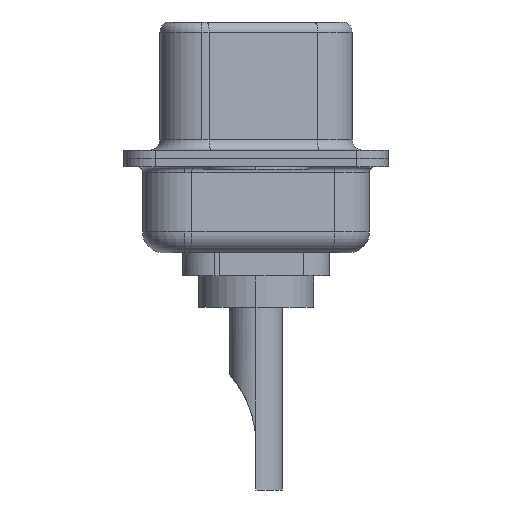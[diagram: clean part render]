
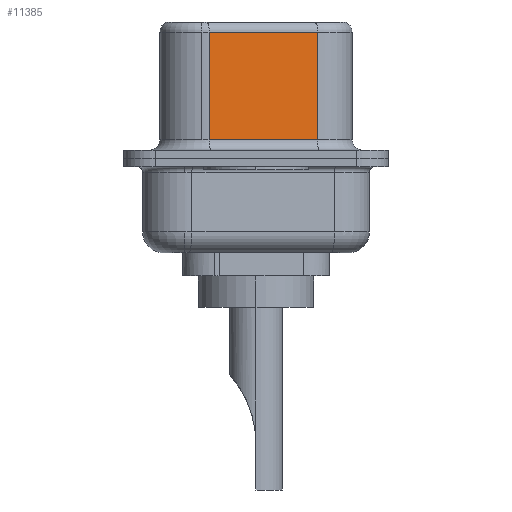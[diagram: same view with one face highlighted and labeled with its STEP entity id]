
A CAD part, left-side view. The second image highlights one B-rep face of the part: STEP entity #11385.
In plain terms, the highlighted planar face has unit normal (-0.985, -0.174, 0).
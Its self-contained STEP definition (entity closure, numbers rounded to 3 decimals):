
#25 = CARTESIAN_POINT ( 'NONE',  ( 4.585, -2.927, 6.02 ) ) ;
#292 = ORIENTED_EDGE ( 'NONE', *, *, #6385, .T. ) ;
#696 = AXIS2_PLACEMENT_3D ( 'NONE', #10534, #4823, #11581 ) ;
#2367 = CARTESIAN_POINT ( 'NONE',  ( 4.585, -2.927, 6.02 ) ) ;
#3522 = DIRECTION ( 'NONE',  ( 0., 0., -1. ) ) ;
#3869 = PLANE ( 'NONE',  #696 ) ;
#4011 = CARTESIAN_POINT ( 'NONE',  ( 3.675, 2.233, 6.52 ) ) ;
#4199 = VECTOR ( 'NONE', #9698, 1000. ) ;
#4581 = CARTESIAN_POINT ( 'NONE',  ( 4.585, -2.927, 0.9 ) ) ;
#4823 = DIRECTION ( 'NONE',  ( 0.985, 0.174, 0. ) ) ;
#4836 = EDGE_LOOP ( 'NONE', ( #8411, #7533, #8234, #292 ) ) ;
#5199 = VERTEX_POINT ( 'NONE', #5674 ) ;
#5299 = VECTOR ( 'NONE', #12026, 1000. ) ;
#5311 = LINE ( 'NONE', #4581, #10063 ) ;
#5546 = VERTEX_POINT ( 'NONE', #5607 ) ;
#5607 = CARTESIAN_POINT ( 'NONE',  ( 3.675, 2.233, 6.02 ) ) ;
#5674 = CARTESIAN_POINT ( 'NONE',  ( 3.675, 2.233, 0.9 ) ) ;
#6385 = EDGE_CURVE ( 'NONE', #5199, #8641, #5311, .T. ) ;
#6741 = LINE ( 'NONE', #4011, #4199 ) ;
#6743 = FACE_OUTER_BOUND ( 'NONE', #4836, .T. ) ;
#6827 = EDGE_CURVE ( 'NONE', #11469, #5546, #7814, .T. ) ;
#7533 = ORIENTED_EDGE ( 'NONE', *, *, #6827, .T. ) ;
#7698 = LINE ( 'NONE', #12219, #10235 ) ;
#7814 = LINE ( 'NONE', #2367, #5299 ) ;
#8059 = EDGE_CURVE ( 'NONE', #5546, #5199, #6741, .T. ) ;
#8234 = ORIENTED_EDGE ( 'NONE', *, *, #8059, .T. ) ;
#8411 = ORIENTED_EDGE ( 'NONE', *, *, #8933, .F. ) ;
#8641 = VERTEX_POINT ( 'NONE', #9727 ) ;
#8933 = EDGE_CURVE ( 'NONE', #11469, #8641, #7698, .T. ) ;
#9698 = DIRECTION ( 'NONE',  ( 0., 0., -1. ) ) ;
#9727 = CARTESIAN_POINT ( 'NONE',  ( 4.585, -2.927, 0.9 ) ) ;
#10063 = VECTOR ( 'NONE', #12091, 1000. ) ;
#10235 = VECTOR ( 'NONE', #3522, 1000. ) ;
#10534 = CARTESIAN_POINT ( 'NONE',  ( 4.585, -2.927, 6.52 ) ) ;
#11385 = ADVANCED_FACE ( 'NONE', ( #6743 ), #3869, .F. ) ;
#11469 = VERTEX_POINT ( 'NONE', #25 ) ;
#11581 = DIRECTION ( 'NONE',  ( -0.174, 0.985, 0. ) ) ;
#12026 = DIRECTION ( 'NONE',  ( -0.174, 0.985, 0. ) ) ;
#12091 = DIRECTION ( 'NONE',  ( 0.174, -0.985, 0. ) ) ;
#12219 = CARTESIAN_POINT ( 'NONE',  ( 4.585, -2.927, 6.52 ) ) ;
